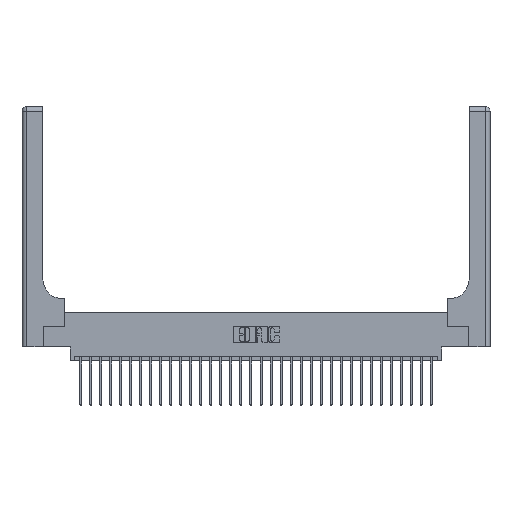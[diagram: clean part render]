
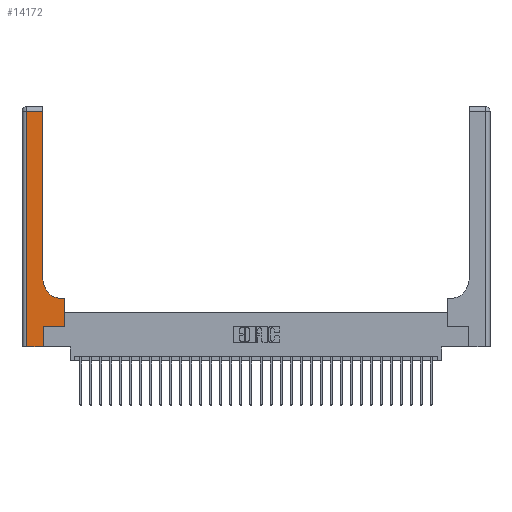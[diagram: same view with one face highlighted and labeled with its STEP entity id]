
A CAD part, top view. The second image highlights one B-rep face of the part: STEP entity #14172.
In plain terms, the highlighted planar face has unit normal (0, 0, 1).
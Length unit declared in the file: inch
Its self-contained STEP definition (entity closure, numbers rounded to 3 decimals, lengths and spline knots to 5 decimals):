
#266 = DIRECTION ( 'NONE',  ( -1., 0., 0. ) ) ;
#553 = ORIENTED_EDGE ( 'NONE', *, *, #21773, .T. ) ;
#567 = LINE ( 'NONE', #14444, #28919 ) ;
#585 = ORIENTED_EDGE ( 'NONE', *, *, #29981, .T. ) ;
#707 = VERTEX_POINT ( 'NONE', #25638 ) ;
#885 = VERTEX_POINT ( 'NONE', #2516 ) ;
#943 = VECTOR ( 'NONE', #18531, 39.37008 ) ;
#1655 = LINE ( 'NONE', #10950, #24758 ) ;
#2516 = CARTESIAN_POINT ( 'NONE',  ( 0.06, 0., 0.37 ) ) ;
#3265 = DIRECTION ( 'NONE',  ( 0., 0., -1. ) ) ;
#4136 = EDGE_CURVE ( 'NONE', #27662, #28351, #4318, .T. ) ;
#4318 = LINE ( 'NONE', #25580, #16623 ) ;
#5168 = LINE ( 'NONE', #5325, #21221 ) ;
#5325 = CARTESIAN_POINT ( 'NONE',  ( 0.26, 0.6, 0.37 ) ) ;
#7086 = EDGE_CURVE ( 'NONE', #14816, #707, #13180, .T. ) ;
#7236 = PLANE ( 'NONE',  #21634 ) ;
#7413 = VERTEX_POINT ( 'NONE', #17563 ) ;
#7659 = LINE ( 'NONE', #14053, #17442 ) ;
#7688 = DIRECTION ( 'NONE',  ( -1., 0., 0. ) ) ;
#8095 = EDGE_CURVE ( 'NONE', #15993, #14816, #19716, .T. ) ;
#8565 = AXIS2_PLACEMENT_3D ( 'NONE', #29824, #15688, #11404 ) ;
#10887 = CARTESIAN_POINT ( 'NONE',  ( 0.26, 3., 0.37 ) ) ;
#10950 = CARTESIAN_POINT ( 'NONE',  ( 0., 2.94, 0.37 ) ) ;
#11404 = DIRECTION ( 'NONE',  ( 1., 0., 0. ) ) ;
#11604 = DIRECTION ( 'NONE',  ( 0., 1., 0. ) ) ;
#11927 = EDGE_CURVE ( 'NONE', #7413, #29905, #567, .T. ) ;
#11980 = CARTESIAN_POINT ( 'NONE',  ( 0.265, 0.25, 0.37 ) ) ;
#13180 = LINE ( 'NONE', #10887, #27145 ) ;
#13423 = CARTESIAN_POINT ( 'NONE',  ( 0.26, 0.85, 0.37 ) ) ;
#14053 = CARTESIAN_POINT ( 'NONE',  ( 0., 0., 0.37 ) ) ;
#14172 = ADVANCED_FACE ( 'NONE', ( #19216 ), #7236, .F. ) ;
#14240 = CARTESIAN_POINT ( 'NONE',  ( 0., 3., 0.37 ) ) ;
#14444 = CARTESIAN_POINT ( 'NONE',  ( 0.265, 0., 0.37 ) ) ;
#14502 = DIRECTION ( 'NONE',  ( 1., 0., 0. ) ) ;
#14816 = VERTEX_POINT ( 'NONE', #13423 ) ;
#15688 = DIRECTION ( 'NONE',  ( 0., 0., -1. ) ) ;
#15993 = VERTEX_POINT ( 'NONE', #19411 ) ;
#16623 = VECTOR ( 'NONE', #11604, 39.37008 ) ;
#17442 = VECTOR ( 'NONE', #14502, 39.37008 ) ;
#17563 = CARTESIAN_POINT ( 'NONE',  ( 0.265, 0., 0.37 ) ) ;
#17802 = ORIENTED_EDGE ( 'NONE', *, *, #8095, .T. ) ;
#18531 = DIRECTION ( 'NONE',  ( 0., -1., 0. ) ) ;
#18671 = LINE ( 'NONE', #25831, #943 ) ;
#19216 = FACE_OUTER_BOUND ( 'NONE', #21309, .T. ) ;
#19411 = CARTESIAN_POINT ( 'NONE',  ( 0.51, 0.6, 0.37 ) ) ;
#19416 = CARTESIAN_POINT ( 'NONE',  ( 0.265, 0.25, 0.37 ) ) ;
#19666 = EDGE_CURVE ( 'NONE', #885, #7413, #7659, .T. ) ;
#19716 = CIRCLE ( 'NONE', #8565, 0.25 ) ;
#19900 = CARTESIAN_POINT ( 'NONE',  ( 0.528, 0.6, 0.37 ) ) ;
#20150 = DIRECTION ( 'NONE',  ( 0., 1., 0. ) ) ;
#20298 = ORIENTED_EDGE ( 'NONE', *, *, #19666, .T. ) ;
#20447 = ORIENTED_EDGE ( 'NONE', *, *, #4136, .T. ) ;
#20651 = ORIENTED_EDGE ( 'NONE', *, *, #11927, .T. ) ;
#20826 = CARTESIAN_POINT ( 'NONE',  ( 0.06, 2.94, 0.37 ) ) ;
#21099 = DIRECTION ( 'NONE',  ( 1., 0., 0. ) ) ;
#21221 = VECTOR ( 'NONE', #266, 39.37008 ) ;
#21309 = EDGE_LOOP ( 'NONE', ( #26246, #29950, #553, #20298, #20651, #585, #20447, #25712, #17802 ) ) ;
#21634 = AXIS2_PLACEMENT_3D ( 'NONE', #14240, #3265, #7688 ) ;
#21687 = EDGE_CURVE ( 'NONE', #707, #25865, #1655, .T. ) ;
#21773 = EDGE_CURVE ( 'NONE', #25865, #885, #18671, .T. ) ;
#24116 = LINE ( 'NONE', #19416, #25707 ) ;
#24758 = VECTOR ( 'NONE', #28267, 39.37008 ) ;
#25580 = CARTESIAN_POINT ( 'NONE',  ( 0.528, 0.25, 0.37 ) ) ;
#25638 = CARTESIAN_POINT ( 'NONE',  ( 0.26, 2.94, 0.37 ) ) ;
#25707 = VECTOR ( 'NONE', #21099, 39.37008 ) ;
#25712 = ORIENTED_EDGE ( 'NONE', *, *, #28169, .T. ) ;
#25741 = CARTESIAN_POINT ( 'NONE',  ( 0.528, 0.25, 0.37 ) ) ;
#25831 = CARTESIAN_POINT ( 'NONE',  ( 0.06, 3., 0.37 ) ) ;
#25865 = VERTEX_POINT ( 'NONE', #20826 ) ;
#26246 = ORIENTED_EDGE ( 'NONE', *, *, #7086, .T. ) ;
#27145 = VECTOR ( 'NONE', #20150, 39.37008 ) ;
#27662 = VERTEX_POINT ( 'NONE', #25741 ) ;
#28130 = DIRECTION ( 'NONE',  ( 0., 1., 0. ) ) ;
#28169 = EDGE_CURVE ( 'NONE', #28351, #15993, #5168, .T. ) ;
#28267 = DIRECTION ( 'NONE',  ( -1., 0., 0. ) ) ;
#28351 = VERTEX_POINT ( 'NONE', #19900 ) ;
#28919 = VECTOR ( 'NONE', #28130, 39.37008 ) ;
#29824 = CARTESIAN_POINT ( 'NONE',  ( 0.51, 0.85, 0.37 ) ) ;
#29905 = VERTEX_POINT ( 'NONE', #11980 ) ;
#29950 = ORIENTED_EDGE ( 'NONE', *, *, #21687, .T. ) ;
#29981 = EDGE_CURVE ( 'NONE', #29905, #27662, #24116, .T. ) ;
